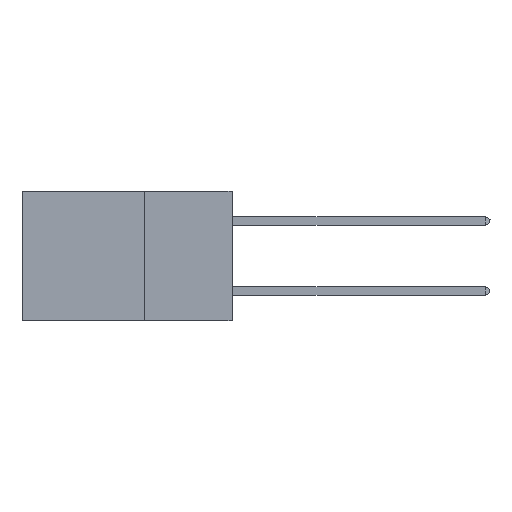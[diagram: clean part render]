
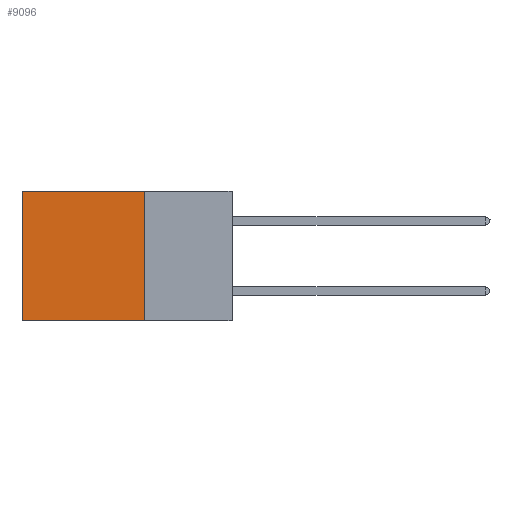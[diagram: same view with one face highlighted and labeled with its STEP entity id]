
A CAD part, left-side view. The second image highlights one B-rep face of the part: STEP entity #9096.
In plain terms, the highlighted planar face has unit normal (-1, 0, 0).
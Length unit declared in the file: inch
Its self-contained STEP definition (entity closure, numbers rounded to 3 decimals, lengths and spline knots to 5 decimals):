
#296 = VECTOR ( 'NONE', #19851, 39.37008 ) ;
#1480 = PLANE ( 'NONE',  #29226 ) ;
#3483 = LINE ( 'NONE', #22797, #27852 ) ;
#3559 = ORIENTED_EDGE ( 'NONE', *, *, #29776, .F. ) ;
#3735 = VERTEX_POINT ( 'NONE', #24502 ) ;
#4317 = EDGE_LOOP ( 'NONE', ( #32199, #23943, #3559, #13948 ) ) ;
#4689 = VERTEX_POINT ( 'NONE', #21460 ) ;
#6252 = DIRECTION ( 'NONE',  ( 0., 1., 0. ) ) ;
#7005 = VERTEX_POINT ( 'NONE', #36032 ) ;
#7682 = EDGE_CURVE ( 'NONE', #3735, #23022, #3483, .T. ) ;
#9096 = ADVANCED_FACE ( 'NONE', ( #35268 ), #1480, .F. ) ;
#9814 = LINE ( 'NONE', #31696, #34302 ) ;
#11488 = DIRECTION ( 'NONE',  ( 0., 0., -1. ) ) ;
#12302 = DIRECTION ( 'NONE',  ( 1., 0., 0. ) ) ;
#13948 = ORIENTED_EDGE ( 'NONE', *, *, #17663, .T. ) ;
#14236 = LINE ( 'NONE', #34070, #14344 ) ;
#14344 = VECTOR ( 'NONE', #6252, 39.37008 ) ;
#15016 = DIRECTION ( 'NONE',  ( 0., 1., 0. ) ) ;
#15991 = DIRECTION ( 'NONE',  ( 0., 0., -1. ) ) ;
#17663 = EDGE_CURVE ( 'NONE', #4689, #3735, #9814, .T. ) ;
#18812 = LINE ( 'NONE', #22990, #296 ) ;
#19851 = DIRECTION ( 'NONE',  ( 0., 0., -1. ) ) ;
#20631 = EDGE_CURVE ( 'NONE', #7005, #23022, #14236, .T. ) ;
#21460 = CARTESIAN_POINT ( 'NONE',  ( 0.2875, 0.25, 0. ) ) ;
#22797 = CARTESIAN_POINT ( 'NONE',  ( 0.2875, 0.6, 0. ) ) ;
#22990 = CARTESIAN_POINT ( 'NONE',  ( 0.2875, 0.25, 0. ) ) ;
#23022 = VERTEX_POINT ( 'NONE', #31655 ) ;
#23943 = ORIENTED_EDGE ( 'NONE', *, *, #20631, .F. ) ;
#24502 = CARTESIAN_POINT ( 'NONE',  ( 0.2875, 0.6, 0. ) ) ;
#27852 = VECTOR ( 'NONE', #11488, 39.37008 ) ;
#29226 = AXIS2_PLACEMENT_3D ( 'NONE', #35081, #12302, #15991 ) ;
#29776 = EDGE_CURVE ( 'NONE', #4689, #7005, #18812, .T. ) ;
#31655 = CARTESIAN_POINT ( 'NONE',  ( 0.2875, 0.6, -0.37 ) ) ;
#31696 = CARTESIAN_POINT ( 'NONE',  ( 0.2875, 0.25, 0. ) ) ;
#32199 = ORIENTED_EDGE ( 'NONE', *, *, #7682, .T. ) ;
#34070 = CARTESIAN_POINT ( 'NONE',  ( 0.2875, 0.25, -0.37 ) ) ;
#34302 = VECTOR ( 'NONE', #15016, 39.37008 ) ;
#35081 = CARTESIAN_POINT ( 'NONE',  ( 0.2875, 0.25, 0. ) ) ;
#35268 = FACE_OUTER_BOUND ( 'NONE', #4317, .T. ) ;
#36032 = CARTESIAN_POINT ( 'NONE',  ( 0.2875, 0.25, -0.37 ) ) ;
